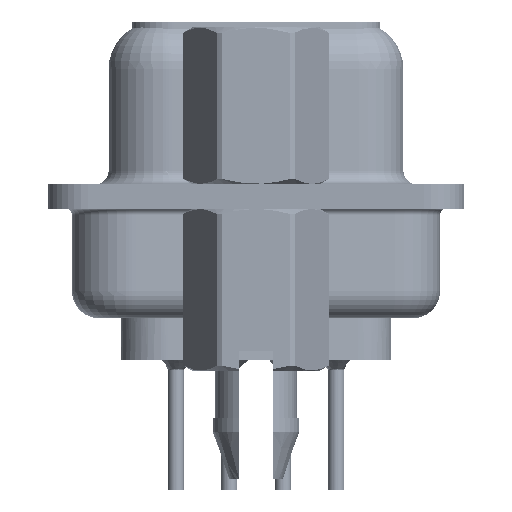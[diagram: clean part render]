
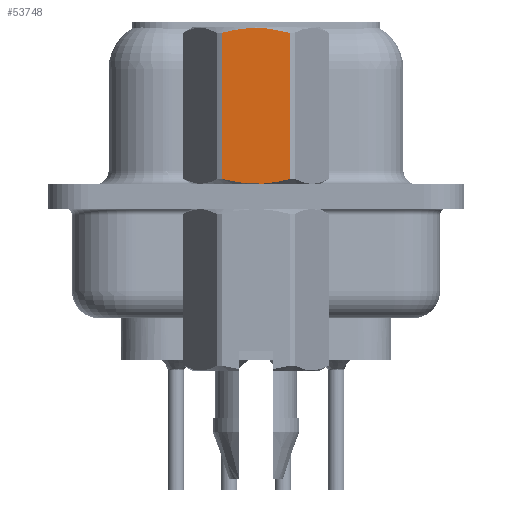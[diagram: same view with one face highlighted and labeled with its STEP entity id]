
A CAD part, left-side view. The second image highlights one B-rep face of the part: STEP entity #53748.
In plain terms, the highlighted planar face has unit normal (-1, 0, 0).
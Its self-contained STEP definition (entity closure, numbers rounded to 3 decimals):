
#246 = FACE_OUTER_BOUND ( 'NONE', #58327, .T. ) ;
#710 = CARTESIAN_POINT ( 'NONE',  ( -2.381, 1.273, 0.652 ) ) ;
#1306 = ORIENTED_EDGE ( 'NONE', *, *, #52058, .T. ) ;
#1933 = EDGE_CURVE ( 'NONE', #34967, #18657, #13197, .T. ) ;
#8795 = CARTESIAN_POINT ( 'NONE',  ( -2.381, -0.858, 6.15 ) ) ;
#10075 = CARTESIAN_POINT ( 'NONE',  ( -2.381, 0.428, 6.215 ) ) ;
#10438 = B_SPLINE_CURVE_WITH_KNOTS ( 'NONE', 3,
 ( #54160, #49008, #29280, #63219, #38992, #33816, #52893, #24102, #43844, #24425 ),
 .UNSPECIFIED., .F., .F.,
 ( 4, 2, 2, 2, 4 ),
 ( 0.003, 0.003, 0.004, 0.004, 0.005 ),
 .UNSPECIFIED. ) ;
#12548 = ORIENTED_EDGE ( 'NONE', *, *, #43992, .T. ) ;
#12714 = EDGE_CURVE ( 'NONE', #18657, #19051, #62243, .T. ) ;
#13197 = LINE ( 'NONE', #32904, #55910 ) ;
#14278 = CARTESIAN_POINT ( 'NONE',  ( -2.381, 1.273, 6.048 ) ) ;
#17021 = VECTOR ( 'NONE', #52483, 1000. ) ;
#18209 = CARTESIAN_POINT ( 'NONE',  ( -2.381, 1.273, 3.792 ) ) ;
#18355 = DIRECTION ( 'NONE',  ( 0., 0., 1. ) ) ;
#18471 = CARTESIAN_POINT ( 'NONE',  ( -2.381, 1.065, 6.104 ) ) ;
#18657 = VERTEX_POINT ( 'NONE', #38891 ) ;
#18803 = CARTESIAN_POINT ( 'NONE',  ( -2.381, 0.215, 6.232 ) ) ;
#19051 = VERTEX_POINT ( 'NONE', #33635 ) ;
#19909 = PLANE ( 'NONE',  #44093 ) ;
#21890 = VERTEX_POINT ( 'NONE', #710 ) ;
#24102 = CARTESIAN_POINT ( 'NONE',  ( -2.381, -0.858, 0.55 ) ) ;
#24425 = CARTESIAN_POINT ( 'NONE',  ( -2.381, -1.273, 0.652 ) ) ;
#29128 = CARTESIAN_POINT ( 'NONE',  ( -2.381, -0.432, 6.215 ) ) ;
#29280 = CARTESIAN_POINT ( 'NONE',  ( -2.381, 0.853, 0.549 ) ) ;
#32904 = CARTESIAN_POINT ( 'NONE',  ( -2.381, -1.273, 3.792 ) ) ;
#33635 = CARTESIAN_POINT ( 'NONE',  ( -2.381, 1.273, 6.048 ) ) ;
#33816 = CARTESIAN_POINT ( 'NONE',  ( -2.381, -0.215, 0.468 ) ) ;
#34967 = VERTEX_POINT ( 'NONE', #57453 ) ;
#35020 = ORIENTED_EDGE ( 'NONE', *, *, #1933, .T. ) ;
#38840 = CARTESIAN_POINT ( 'NONE',  ( -2.381, -1.273, 6.048 ) ) ;
#38891 = CARTESIAN_POINT ( 'NONE',  ( -2.381, -1.273, 6.048 ) ) ;
#38992 = CARTESIAN_POINT ( 'NONE',  ( -2.381, 0.215, 0.468 ) ) ;
#39633 = DIRECTION ( 'NONE',  ( 0., -1., 0. ) ) ;
#43112 = LINE ( 'NONE', #18209, #17021 ) ;
#43515 = CARTESIAN_POINT ( 'NONE',  ( -2.381, 1.375, -3.75 ) ) ;
#43844 = CARTESIAN_POINT ( 'NONE',  ( -2.381, -1.066, 0.596 ) ) ;
#43992 = EDGE_CURVE ( 'NONE', #21890, #34967, #10438, .T. ) ;
#44093 = AXIS2_PLACEMENT_3D ( 'NONE', #43515, #63216, #39633 ) ;
#45058 = ORIENTED_EDGE ( 'NONE', *, *, #12714, .T. ) ;
#48220 = CARTESIAN_POINT ( 'NONE',  ( -2.381, 0.853, 6.151 ) ) ;
#49008 = CARTESIAN_POINT ( 'NONE',  ( -2.381, 1.065, 0.596 ) ) ;
#52058 = EDGE_CURVE ( 'NONE', #19051, #21890, #43112, .T. ) ;
#52483 = DIRECTION ( 'NONE',  ( 0., 0., -1. ) ) ;
#52893 = CARTESIAN_POINT ( 'NONE',  ( -2.381, -0.432, 0.485 ) ) ;
#53748 = ADVANCED_FACE ( 'NONE', ( #246 ), #19909, .T. ) ;
#54160 = CARTESIAN_POINT ( 'NONE',  ( -2.381, 1.273, 0.652 ) ) ;
#54345 = CARTESIAN_POINT ( 'NONE',  ( -2.381, -0.215, 6.232 ) ) ;
#55910 = VECTOR ( 'NONE', #18355, 1000. ) ;
#57453 = CARTESIAN_POINT ( 'NONE',  ( -2.381, -1.273, 0.652 ) ) ;
#58327 = EDGE_LOOP ( 'NONE', ( #12548, #35020, #45058, #1306 ) ) ;
#62243 = B_SPLINE_CURVE_WITH_KNOTS ( 'NONE', 3,
 ( #38840, #62746, #8795, #29128, #54345, #18803, #10075, #48220, #18471, #14278 ),
 .UNSPECIFIED., .F., .F.,
 ( 4, 2, 2, 2, 4 ),
 ( 0.001, 0.002, 0.002, 0.003, 0.004 ),
 .UNSPECIFIED. ) ;
#62746 = CARTESIAN_POINT ( 'NONE',  ( -2.381, -1.066, 6.104 ) ) ;
#63216 = DIRECTION ( 'NONE',  ( -1., 0., 0. ) ) ;
#63219 = CARTESIAN_POINT ( 'NONE',  ( -2.381, 0.428, 0.485 ) ) ;
